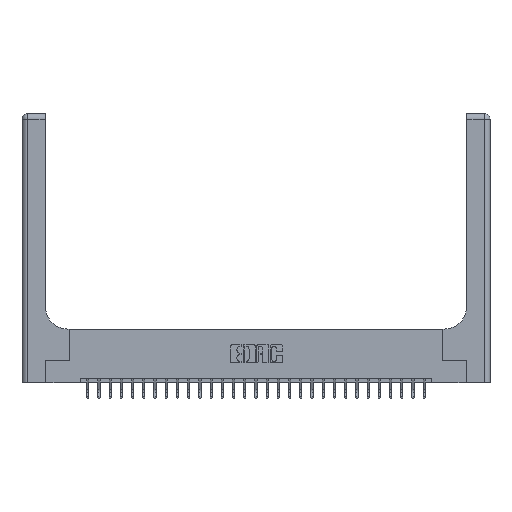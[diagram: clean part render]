
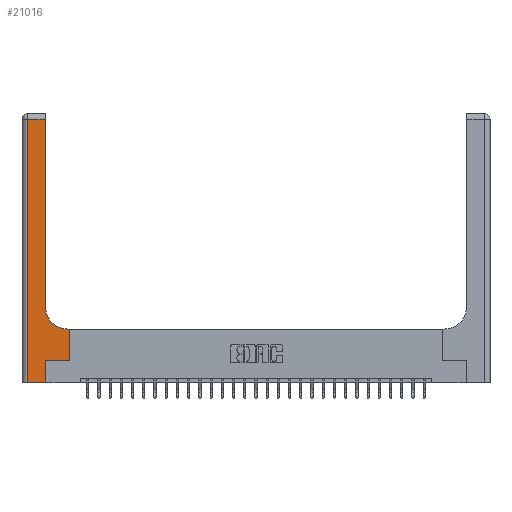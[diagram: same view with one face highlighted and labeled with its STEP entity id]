
A CAD part, top view. The second image highlights one B-rep face of the part: STEP entity #21016.
In plain terms, the highlighted planar face has unit normal (0, 0, 1).
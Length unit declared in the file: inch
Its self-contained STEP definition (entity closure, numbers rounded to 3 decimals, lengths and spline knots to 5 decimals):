
#115 = DIRECTION ( 'NONE',  ( 0., 0., -1. ) ) ;
#658 = PLANE ( 'NONE',  #16490 ) ;
#826 = EDGE_CURVE ( 'NONE', #9905, #7372, #18616, .T. ) ;
#1049 = VERTEX_POINT ( 'NONE', #11172 ) ;
#1140 = DIRECTION ( 'NONE',  ( 1., 0., 0. ) ) ;
#1256 = EDGE_CURVE ( 'NONE', #11181, #3657, #26945, .T. ) ;
#1526 = LINE ( 'NONE', #22999, #6606 ) ;
#2061 = CARTESIAN_POINT ( 'NONE',  ( 0.26, 2.94, 0.37 ) ) ;
#2337 = CARTESIAN_POINT ( 'NONE',  ( 0.26, 0.6, 0.37 ) ) ;
#2684 = LINE ( 'NONE', #13554, #19992 ) ;
#3312 = ORIENTED_EDGE ( 'NONE', *, *, #8610, .T. ) ;
#3363 = VECTOR ( 'NONE', #17805, 39.37008 ) ;
#3376 = VERTEX_POINT ( 'NONE', #12417 ) ;
#3399 = LINE ( 'NONE', #11904, #7732 ) ;
#3657 = VERTEX_POINT ( 'NONE', #20351 ) ;
#3804 = CARTESIAN_POINT ( 'NONE',  ( 0.265, 0.25, 0.37 ) ) ;
#3928 = DIRECTION ( 'NONE',  ( 1., 0., 0. ) ) ;
#5537 = VERTEX_POINT ( 'NONE', #3804 ) ;
#5589 = CARTESIAN_POINT ( 'NONE',  ( 0., 0., 0.37 ) ) ;
#5606 = ORIENTED_EDGE ( 'NONE', *, *, #20165, .T. ) ;
#5736 = CARTESIAN_POINT ( 'NONE',  ( 0.06, 0., 0.37 ) ) ;
#6606 = VECTOR ( 'NONE', #12386, 39.37008 ) ;
#6923 = FACE_OUTER_BOUND ( 'NONE', #18530, .T. ) ;
#7372 = VERTEX_POINT ( 'NONE', #2061 ) ;
#7732 = VECTOR ( 'NONE', #16262, 39.37008 ) ;
#8360 = CARTESIAN_POINT ( 'NONE',  ( 0.26, 0.85, 0.37 ) ) ;
#8610 = EDGE_CURVE ( 'NONE', #9823, #11181, #22747, .T. ) ;
#9797 = ORIENTED_EDGE ( 'NONE', *, *, #27487, .T. ) ;
#9823 = VERTEX_POINT ( 'NONE', #16215 ) ;
#9905 = VERTEX_POINT ( 'NONE', #8360 ) ;
#10678 = EDGE_CURVE ( 'NONE', #3376, #11443, #3399, .T. ) ;
#10963 = AXIS2_PLACEMENT_3D ( 'NONE', #20826, #16660, #3928 ) ;
#10978 = ORIENTED_EDGE ( 'NONE', *, *, #19659, .T. ) ;
#11039 = DIRECTION ( 'NONE',  ( -1., 0., 0. ) ) ;
#11102 = ORIENTED_EDGE ( 'NONE', *, *, #10678, .T. ) ;
#11162 = ORIENTED_EDGE ( 'NONE', *, *, #826, .T. ) ;
#11172 = CARTESIAN_POINT ( 'NONE',  ( 0.51, 0.6, 0.37 ) ) ;
#11181 = VERTEX_POINT ( 'NONE', #5736 ) ;
#11443 = VERTEX_POINT ( 'NONE', #17591 ) ;
#11904 = CARTESIAN_POINT ( 'NONE',  ( 0.528, 0.25, 0.37 ) ) ;
#12386 = DIRECTION ( 'NONE',  ( 0., 1., 0. ) ) ;
#12417 = CARTESIAN_POINT ( 'NONE',  ( 0.528, 0.25, 0.37 ) ) ;
#12558 = VECTOR ( 'NONE', #20928, 39.37008 ) ;
#12678 = CARTESIAN_POINT ( 'NONE',  ( 0.06, 3., 0.37 ) ) ;
#13285 = ORIENTED_EDGE ( 'NONE', *, *, #15357, .T. ) ;
#13554 = CARTESIAN_POINT ( 'NONE',  ( 0., 2.94, 0.37 ) ) ;
#14096 = CIRCLE ( 'NONE', #10963, 0.25 ) ;
#14488 = EDGE_CURVE ( 'NONE', #11443, #1049, #26307, .T. ) ;
#15043 = CARTESIAN_POINT ( 'NONE',  ( 0., 3., 0.37 ) ) ;
#15357 = EDGE_CURVE ( 'NONE', #1049, #9905, #14096, .T. ) ;
#16215 = CARTESIAN_POINT ( 'NONE',  ( 0.06, 2.94, 0.37 ) ) ;
#16262 = DIRECTION ( 'NONE',  ( 0., 1., 0. ) ) ;
#16490 = AXIS2_PLACEMENT_3D ( 'NONE', #15043, #115, #21599 ) ;
#16660 = DIRECTION ( 'NONE',  ( 0., 0., -1. ) ) ;
#17591 = CARTESIAN_POINT ( 'NONE',  ( 0.528, 0.6, 0.37 ) ) ;
#17805 = DIRECTION ( 'NONE',  ( -1., 0., 0. ) ) ;
#17885 = CARTESIAN_POINT ( 'NONE',  ( 0.265, 0.25, 0.37 ) ) ;
#18530 = EDGE_LOOP ( 'NONE', ( #11162, #5606, #3312, #19236, #10978, #9797, #11102, #20262, #13285 ) ) ;
#18616 = LINE ( 'NONE', #25175, #18843 ) ;
#18843 = VECTOR ( 'NONE', #22525, 39.37008 ) ;
#19216 = DIRECTION ( 'NONE',  ( 1., 0., 0. ) ) ;
#19236 = ORIENTED_EDGE ( 'NONE', *, *, #1256, .T. ) ;
#19659 = EDGE_CURVE ( 'NONE', #3657, #5537, #1526, .T. ) ;
#19992 = VECTOR ( 'NONE', #11039, 39.37008 ) ;
#20165 = EDGE_CURVE ( 'NONE', #7372, #9823, #2684, .T. ) ;
#20262 = ORIENTED_EDGE ( 'NONE', *, *, #14488, .T. ) ;
#20351 = CARTESIAN_POINT ( 'NONE',  ( 0.265, 0., 0.37 ) ) ;
#20826 = CARTESIAN_POINT ( 'NONE',  ( 0.51, 0.85, 0.37 ) ) ;
#20928 = DIRECTION ( 'NONE',  ( 0., -1., 0. ) ) ;
#21016 = ADVANCED_FACE ( 'NONE', ( #6923 ), #658, .F. ) ;
#21599 = DIRECTION ( 'NONE',  ( -1., 0., 0. ) ) ;
#22525 = DIRECTION ( 'NONE',  ( 0., 1., 0. ) ) ;
#22747 = LINE ( 'NONE', #12678, #12558 ) ;
#22888 = VECTOR ( 'NONE', #1140, 39.37008 ) ;
#22999 = CARTESIAN_POINT ( 'NONE',  ( 0.265, 0., 0.37 ) ) ;
#23256 = LINE ( 'NONE', #17885, #26744 ) ;
#25175 = CARTESIAN_POINT ( 'NONE',  ( 0.26, 3., 0.37 ) ) ;
#26307 = LINE ( 'NONE', #2337, #3363 ) ;
#26744 = VECTOR ( 'NONE', #19216, 39.37008 ) ;
#26945 = LINE ( 'NONE', #5589, #22888 ) ;
#27487 = EDGE_CURVE ( 'NONE', #5537, #3376, #23256, .T. ) ;
